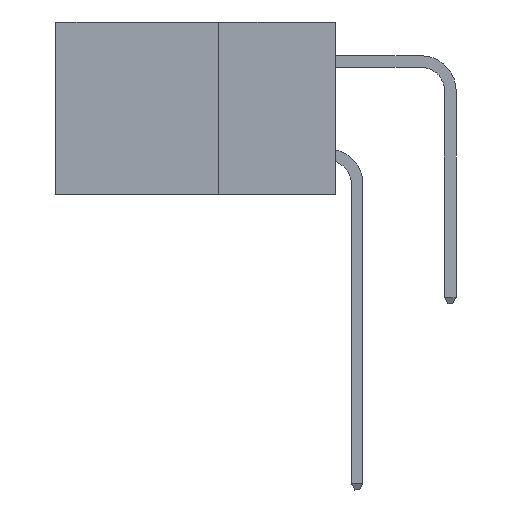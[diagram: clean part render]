
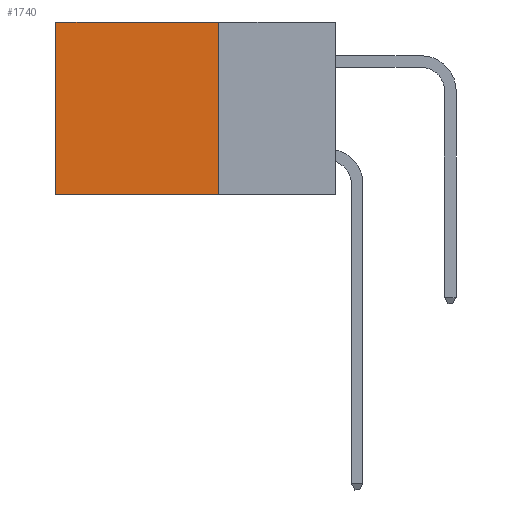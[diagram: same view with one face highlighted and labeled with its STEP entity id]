
A CAD part, left-side view. The second image highlights one B-rep face of the part: STEP entity #1740.
In plain terms, the highlighted planar face has unit normal (-1, 0, 0).
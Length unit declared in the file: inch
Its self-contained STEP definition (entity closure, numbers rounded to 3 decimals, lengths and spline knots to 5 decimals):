
#109 = LINE ( 'NONE', #5359, #10520 ) ;
#775 = CARTESIAN_POINT ( 'NONE',  ( 0.2875, 0.25, -0.37 ) ) ;
#1292 = VERTEX_POINT ( 'NONE', #11107 ) ;
#1330 = VECTOR ( 'NONE', #12978, 39.37008 ) ;
#1483 = VERTEX_POINT ( 'NONE', #9363 ) ;
#1633 = DIRECTION ( 'NONE',  ( 0., 0., -1. ) ) ;
#1740 = ADVANCED_FACE ( 'NONE', ( #13396 ), #3900, .F. ) ;
#1992 = LINE ( 'NONE', #9664, #8164 ) ;
#2164 = AXIS2_PLACEMENT_3D ( 'NONE', #8608, #8654, #1633 ) ;
#2494 = CARTESIAN_POINT ( 'NONE',  ( 0.2875, 0.25, 0. ) ) ;
#3057 = CARTESIAN_POINT ( 'NONE',  ( 0.2875, 0.25, 0. ) ) ;
#3900 = PLANE ( 'NONE',  #2164 ) ;
#3939 = VERTEX_POINT ( 'NONE', #775 ) ;
#4262 = ORIENTED_EDGE ( 'NONE', *, *, #10994, .F. ) ;
#5257 = DIRECTION ( 'NONE',  ( 0., 0., -1. ) ) ;
#5359 = CARTESIAN_POINT ( 'NONE',  ( 0.2875, 0.6, 0. ) ) ;
#6994 = ORIENTED_EDGE ( 'NONE', *, *, #12168, .T. ) ;
#7580 = EDGE_CURVE ( 'NONE', #3939, #1483, #1992, .T. ) ;
#8164 = VECTOR ( 'NONE', #8656, 39.37008 ) ;
#8608 = CARTESIAN_POINT ( 'NONE',  ( 0.2875, 0.25, 0. ) ) ;
#8654 = DIRECTION ( 'NONE',  ( 1., 0., 0. ) ) ;
#8656 = DIRECTION ( 'NONE',  ( 0., 1., 0. ) ) ;
#9363 = CARTESIAN_POINT ( 'NONE',  ( 0.2875, 0.6, -0.37 ) ) ;
#9413 = EDGE_CURVE ( 'NONE', #12844, #1292, #13402, .T. ) ;
#9664 = CARTESIAN_POINT ( 'NONE',  ( 0.2875, 0.25, -0.37 ) ) ;
#10210 = EDGE_LOOP ( 'NONE', ( #6994, #10716, #4262, #12522 ) ) ;
#10520 = VECTOR ( 'NONE', #5257, 39.37008 ) ;
#10716 = ORIENTED_EDGE ( 'NONE', *, *, #7580, .F. ) ;
#10994 = EDGE_CURVE ( 'NONE', #12844, #3939, #11355, .T. ) ;
#11107 = CARTESIAN_POINT ( 'NONE',  ( 0.2875, 0.6, 0. ) ) ;
#11355 = LINE ( 'NONE', #14125, #1330 ) ;
#11603 = DIRECTION ( 'NONE',  ( 0., 1., 0. ) ) ;
#12145 = VECTOR ( 'NONE', #11603, 39.37008 ) ;
#12168 = EDGE_CURVE ( 'NONE', #1292, #1483, #109, .T. ) ;
#12522 = ORIENTED_EDGE ( 'NONE', *, *, #9413, .T. ) ;
#12844 = VERTEX_POINT ( 'NONE', #3057 ) ;
#12978 = DIRECTION ( 'NONE',  ( 0., 0., -1. ) ) ;
#13396 = FACE_OUTER_BOUND ( 'NONE', #10210, .T. ) ;
#13402 = LINE ( 'NONE', #2494, #12145 ) ;
#14125 = CARTESIAN_POINT ( 'NONE',  ( 0.2875, 0.25, 0. ) ) ;
